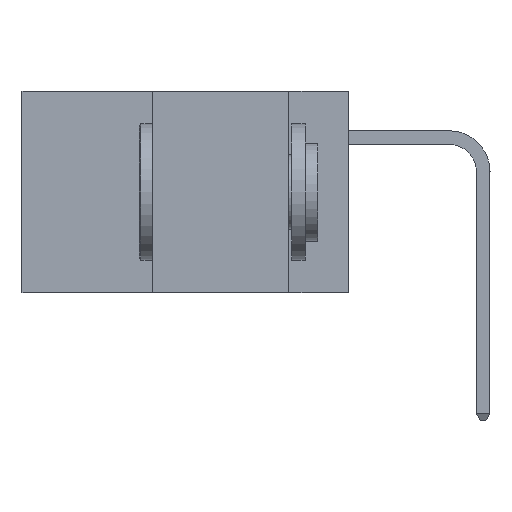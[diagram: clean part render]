
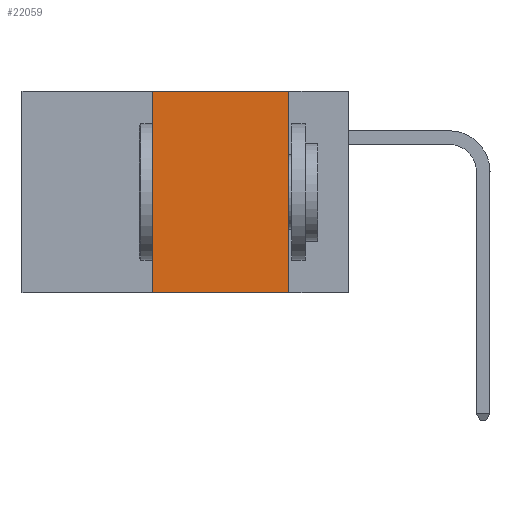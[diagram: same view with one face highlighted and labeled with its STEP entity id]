
A CAD part, left-side view. The second image highlights one B-rep face of the part: STEP entity #22059.
In plain terms, the highlighted planar face has unit normal (-1, 0, 0).
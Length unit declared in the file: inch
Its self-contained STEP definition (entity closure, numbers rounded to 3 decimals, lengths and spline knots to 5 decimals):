
#705 = CARTESIAN_POINT ( 'NONE',  ( 0., 0.36, 0. ) ) ;
#1153 = FACE_OUTER_BOUND ( 'NONE', #7520, .T. ) ;
#1393 = DIRECTION ( 'NONE',  ( 1., 0., 0. ) ) ;
#1580 = ORIENTED_EDGE ( 'NONE', *, *, #19943, .F. ) ;
#2221 = LINE ( 'NONE', #12829, #13008 ) ;
#2923 = ORIENTED_EDGE ( 'NONE', *, *, #6704, .F. ) ;
#5076 = CARTESIAN_POINT ( 'NONE',  ( 0., 0.36, -0.37 ) ) ;
#5885 = CARTESIAN_POINT ( 'NONE',  ( 0., 0.11, -0.37 ) ) ;
#6704 = EDGE_CURVE ( 'NONE', #10910, #18451, #2221, .T. ) ;
#7058 = VECTOR ( 'NONE', #11378, 39.37008 ) ;
#7062 = CARTESIAN_POINT ( 'NONE',  ( 0., 0.6, -0.37 ) ) ;
#7520 = EDGE_LOOP ( 'NONE', ( #1580, #2923, #14342, #16948 ) ) ;
#8145 = EDGE_CURVE ( 'NONE', #23101, #20292, #18275, .T. ) ;
#10910 = VERTEX_POINT ( 'NONE', #705 ) ;
#11378 = DIRECTION ( 'NONE',  ( 0., -1., 0. ) ) ;
#12829 = CARTESIAN_POINT ( 'NONE',  ( 0., 0.6, 0. ) ) ;
#13008 = VECTOR ( 'NONE', #14903, 39.37008 ) ;
#14248 = CARTESIAN_POINT ( 'NONE',  ( 0., 0.6, 0. ) ) ;
#14342 = ORIENTED_EDGE ( 'NONE', *, *, #22183, .F. ) ;
#14595 = CARTESIAN_POINT ( 'NONE',  ( 0., 0.36, 0. ) ) ;
#14903 = DIRECTION ( 'NONE',  ( 0., -1., 0. ) ) ;
#15301 = VECTOR ( 'NONE', #23815, 39.37008 ) ;
#15949 = LINE ( 'NONE', #21670, #15301 ) ;
#16333 = DIRECTION ( 'NONE',  ( 0., 0., -1. ) ) ;
#16923 = AXIS2_PLACEMENT_3D ( 'NONE', #14248, #1393, #16333 ) ;
#16948 = ORIENTED_EDGE ( 'NONE', *, *, #8145, .T. ) ;
#17069 = DIRECTION ( 'NONE',  ( 0., 0., 1. ) ) ;
#18275 = LINE ( 'NONE', #7062, #7058 ) ;
#18451 = VERTEX_POINT ( 'NONE', #18621 ) ;
#18621 = CARTESIAN_POINT ( 'NONE',  ( 0., 0.11, 0. ) ) ;
#19797 = LINE ( 'NONE', #14595, #24762 ) ;
#19943 = EDGE_CURVE ( 'NONE', #18451, #20292, #15949, .T. ) ;
#20292 = VERTEX_POINT ( 'NONE', #5885 ) ;
#21670 = CARTESIAN_POINT ( 'NONE',  ( 0., 0.11, 0. ) ) ;
#22059 = ADVANCED_FACE ( 'NONE', ( #1153 ), #26852, .F. ) ;
#22183 = EDGE_CURVE ( 'NONE', #23101, #10910, #19797, .T. ) ;
#23101 = VERTEX_POINT ( 'NONE', #5076 ) ;
#23815 = DIRECTION ( 'NONE',  ( 0., 0., -1. ) ) ;
#24762 = VECTOR ( 'NONE', #17069, 39.37008 ) ;
#26852 = PLANE ( 'NONE',  #16923 ) ;
